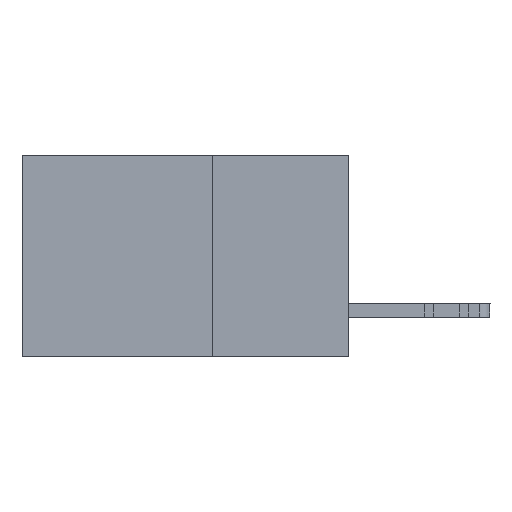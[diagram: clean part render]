
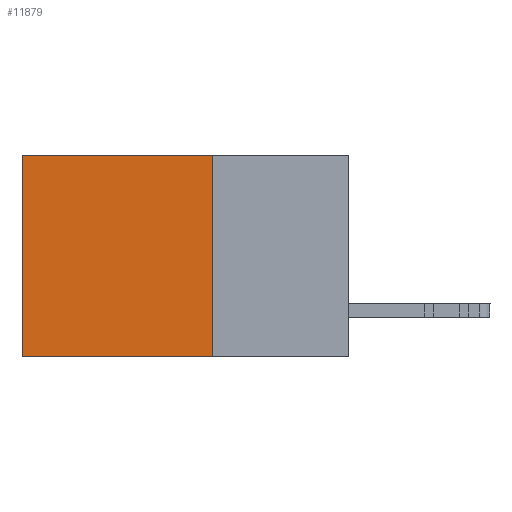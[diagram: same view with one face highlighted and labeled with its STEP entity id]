
A CAD part, left-side view. The second image highlights one B-rep face of the part: STEP entity #11879.
In plain terms, the highlighted planar face has unit normal (-1, 0, 0).
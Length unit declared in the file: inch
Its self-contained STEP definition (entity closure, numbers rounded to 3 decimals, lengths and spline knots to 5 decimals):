
#126 = DIRECTION ( 'NONE',  ( 0., 0., -1. ) ) ;
#2402 = CARTESIAN_POINT ( 'NONE',  ( 0.2615, 0.6, -0.37 ) ) ;
#3995 = ORIENTED_EDGE ( 'NONE', *, *, #6041, .F. ) ;
#4858 = CARTESIAN_POINT ( 'NONE',  ( 0.2615, 0.6, 0. ) ) ;
#5857 = CARTESIAN_POINT ( 'NONE',  ( 0.2615, 0.25, -0.37 ) ) ;
#6041 = EDGE_CURVE ( 'NONE', #18870, #21839, #23694, .T. ) ;
#6126 = VECTOR ( 'NONE', #19158, 39.37008 ) ;
#6597 = CARTESIAN_POINT ( 'NONE',  ( 0.2615, 0.25, -0.37 ) ) ;
#6629 = VERTEX_POINT ( 'NONE', #19515 ) ;
#9212 = CARTESIAN_POINT ( 'NONE',  ( 0.2615, 0.25, 0. ) ) ;
#9885 = AXIS2_PLACEMENT_3D ( 'NONE', #6597, #14498, #22233 ) ;
#10667 = FACE_OUTER_BOUND ( 'NONE', #14471, .T. ) ;
#11094 = VECTOR ( 'NONE', #126, 39.37008 ) ;
#11724 = EDGE_CURVE ( 'NONE', #18489, #21839, #14003, .T. ) ;
#11862 = CARTESIAN_POINT ( 'NONE',  ( 0.2615, 0.6, -0.37 ) ) ;
#11872 = CARTESIAN_POINT ( 'NONE',  ( 0.2615, 0.25, -0.37 ) ) ;
#11879 = ADVANCED_FACE ( 'NONE', ( #10667 ), #18569, .F. ) ;
#14003 = LINE ( 'NONE', #2402, #11094 ) ;
#14471 = EDGE_LOOP ( 'NONE', ( #23466, #3995, #24313, #21971 ) ) ;
#14498 = DIRECTION ( 'NONE',  ( 1., 0., 0. ) ) ;
#17166 = EDGE_CURVE ( 'NONE', #6629, #18870, #23418, .T. ) ;
#17345 = DIRECTION ( 'NONE',  ( 0., 0., -1. ) ) ;
#17862 = CARTESIAN_POINT ( 'NONE',  ( 0.2615, 0.25, -0.37 ) ) ;
#18489 = VERTEX_POINT ( 'NONE', #4858 ) ;
#18569 = PLANE ( 'NONE',  #9885 ) ;
#18870 = VERTEX_POINT ( 'NONE', #5857 ) ;
#19034 = VECTOR ( 'NONE', #23945, 39.37008 ) ;
#19158 = DIRECTION ( 'NONE',  ( 0., 1., 0. ) ) ;
#19515 = CARTESIAN_POINT ( 'NONE',  ( 0.2615, 0.25, 0. ) ) ;
#20796 = LINE ( 'NONE', #9212, #6126 ) ;
#21839 = VERTEX_POINT ( 'NONE', #11862 ) ;
#21971 = ORIENTED_EDGE ( 'NONE', *, *, #24989, .T. ) ;
#22179 = VECTOR ( 'NONE', #17345, 39.37008 ) ;
#22233 = DIRECTION ( 'NONE',  ( 0., 0., -1. ) ) ;
#23418 = LINE ( 'NONE', #11872, #22179 ) ;
#23466 = ORIENTED_EDGE ( 'NONE', *, *, #11724, .T. ) ;
#23694 = LINE ( 'NONE', #17862, #19034 ) ;
#23945 = DIRECTION ( 'NONE',  ( 0., 1., 0. ) ) ;
#24313 = ORIENTED_EDGE ( 'NONE', *, *, #17166, .F. ) ;
#24989 = EDGE_CURVE ( 'NONE', #6629, #18489, #20796, .T. ) ;
